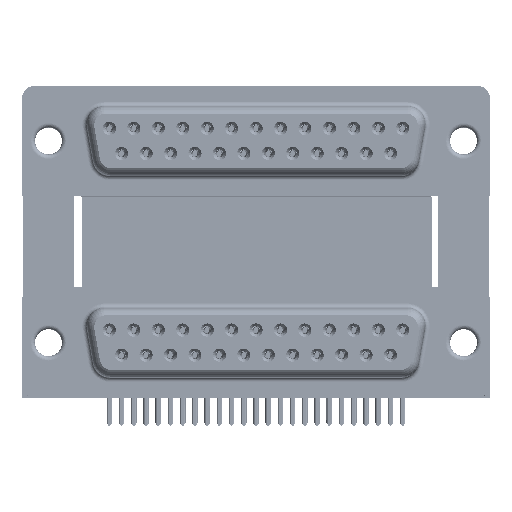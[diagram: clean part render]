
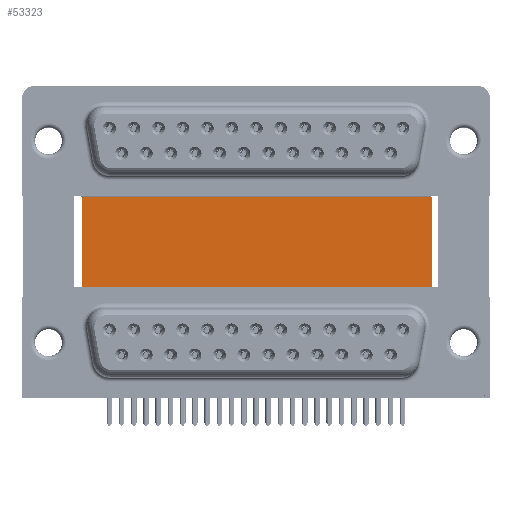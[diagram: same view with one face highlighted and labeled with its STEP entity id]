
A CAD part, top view. The second image highlights one B-rep face of the part: STEP entity #53323.
In plain terms, the highlighted planar face has unit normal (0, 0, 1).
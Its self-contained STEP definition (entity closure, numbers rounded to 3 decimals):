
#3017 = ORIENTED_EDGE ( 'NONE', *, *, #54240, .F. ) ;
#4946 = CARTESIAN_POINT ( 'NONE',  ( 3.79, 16.585, -12. ) ) ;
#7374 = CARTESIAN_POINT ( 'NONE',  ( 3.79, -3.735, -12. ) ) ;
#8183 = VERTEX_POINT ( 'NONE', #12876 ) ;
#11640 = ORIENTED_EDGE ( 'NONE', *, *, #55488, .T. ) ;
#11800 = ORIENTED_EDGE ( 'NONE', *, *, #22989, .T. ) ;
#12100 = VECTOR ( 'NONE', #44757, 1000. ) ;
#12876 = CARTESIAN_POINT ( 'NONE',  ( 3.79, -3.735, -12. ) ) ;
#12911 = DIRECTION ( 'NONE',  ( 0., -1., 0. ) ) ;
#17595 = LINE ( 'NONE', #43450, #24757 ) ;
#18478 = VECTOR ( 'NONE', #21162, 1000. ) ;
#21162 = DIRECTION ( 'NONE',  ( 1., 0., 0. ) ) ;
#22008 = FACE_OUTER_BOUND ( 'NONE', #32715, .T. ) ;
#22989 = EDGE_CURVE ( 'NONE', #27044, #8183, #17595, .T. ) ;
#23386 = EDGE_CURVE ( 'NONE', #27044, #36615, #39485, .T. ) ;
#24757 = VECTOR ( 'NONE', #12911, 1000. ) ;
#25328 = ORIENTED_EDGE ( 'NONE', *, *, #23386, .F. ) ;
#26254 = CARTESIAN_POINT ( 'NONE',  ( 3.79, 16.585, -12. ) ) ;
#26415 = PLANE ( 'NONE',  #51074 ) ;
#26428 = VERTEX_POINT ( 'NONE', #30831 ) ;
#26988 = DIRECTION ( 'NONE',  ( 0., 0., -1. ) ) ;
#27044 = VERTEX_POINT ( 'NONE', #39431 ) ;
#29683 = LINE ( 'NONE', #7374, #18478 ) ;
#30831 = CARTESIAN_POINT ( 'NONE',  ( 43.43, -3.735, -12. ) ) ;
#31391 = DIRECTION ( 'NONE',  ( 0., -1., 0. ) ) ;
#32715 = EDGE_LOOP ( 'NONE', ( #11640, #3017, #25328, #11800 ) ) ;
#36615 = VERTEX_POINT ( 'NONE', #55220 ) ;
#36681 = LINE ( 'NONE', #57827, #40909 ) ;
#39431 = CARTESIAN_POINT ( 'NONE',  ( 3.79, 16.585, -12. ) ) ;
#39485 = LINE ( 'NONE', #26254, #12100 ) ;
#40218 = DIRECTION ( 'NONE',  ( -1., 0., 0. ) ) ;
#40909 = VECTOR ( 'NONE', #31391, 1000. ) ;
#43450 = CARTESIAN_POINT ( 'NONE',  ( 3.79, 16.585, -12. ) ) ;
#44757 = DIRECTION ( 'NONE',  ( 1., 0., 0. ) ) ;
#51074 = AXIS2_PLACEMENT_3D ( 'NONE', #4946, #26988, #40218 ) ;
#53323 = ADVANCED_FACE ( 'NONE', ( #22008 ), #26415, .F. ) ;
#54240 = EDGE_CURVE ( 'NONE', #36615, #26428, #36681, .T. ) ;
#55220 = CARTESIAN_POINT ( 'NONE',  ( 43.43, 16.585, -12. ) ) ;
#55488 = EDGE_CURVE ( 'NONE', #8183, #26428, #29683, .T. ) ;
#57827 = CARTESIAN_POINT ( 'NONE',  ( 43.43, 16.585, -12. ) ) ;
